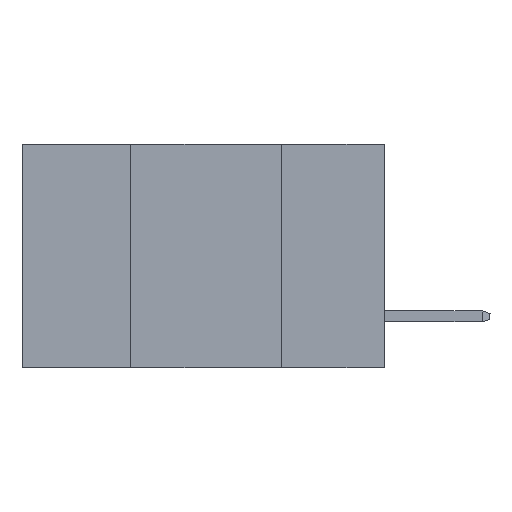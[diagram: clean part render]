
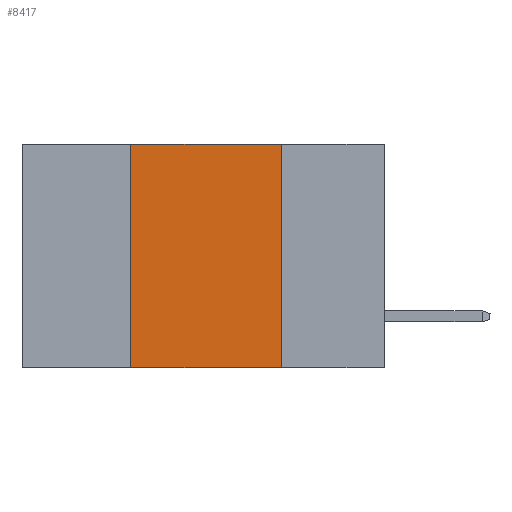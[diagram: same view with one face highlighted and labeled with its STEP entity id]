
A CAD part, left-side view. The second image highlights one B-rep face of the part: STEP entity #8417.
In plain terms, the highlighted planar face has unit normal (-1, 0, 0).
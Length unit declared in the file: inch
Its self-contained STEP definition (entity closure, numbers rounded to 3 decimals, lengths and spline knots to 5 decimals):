
#395 = DIRECTION ( 'NONE',  ( 0., 0., 1. ) ) ;
#570 = LINE ( 'NONE', #4150, #7495 ) ;
#981 = VECTOR ( 'NONE', #5233, 39.37008 ) ;
#1358 = EDGE_CURVE ( 'NONE', #10059, #4949, #4970, .T. ) ;
#1696 = LINE ( 'NONE', #1801, #981 ) ;
#1801 = CARTESIAN_POINT ( 'NONE',  ( 0., 0.6, 0. ) ) ;
#1817 = EDGE_CURVE ( 'NONE', #10059, #9994, #570, .T. ) ;
#1960 = ORIENTED_EDGE ( 'NONE', *, *, #1817, .F. ) ;
#2254 = EDGE_CURVE ( 'NONE', #6924, #4949, #11538, .T. ) ;
#2487 = DIRECTION ( 'NONE',  ( 0., -1., 0. ) ) ;
#2564 = CARTESIAN_POINT ( 'NONE',  ( 0., 0.17, -0.37 ) ) ;
#4150 = CARTESIAN_POINT ( 'NONE',  ( 0., 0.42, -0.37 ) ) ;
#4535 = CARTESIAN_POINT ( 'NONE',  ( 0., 0.42, 0. ) ) ;
#4606 = FACE_OUTER_BOUND ( 'NONE', #9052, .T. ) ;
#4664 = EDGE_CURVE ( 'NONE', #9994, #6924, #1696, .T. ) ;
#4949 = VERTEX_POINT ( 'NONE', #9545 ) ;
#4970 = LINE ( 'NONE', #6088, #8031 ) ;
#5233 = DIRECTION ( 'NONE',  ( 0., -1., 0. ) ) ;
#5314 = PLANE ( 'NONE',  #10304 ) ;
#6088 = CARTESIAN_POINT ( 'NONE',  ( 0., 0.6, -0.37 ) ) ;
#6427 = CARTESIAN_POINT ( 'NONE',  ( 0., 0.42, -0.37 ) ) ;
#6924 = VERTEX_POINT ( 'NONE', #9093 ) ;
#6939 = ORIENTED_EDGE ( 'NONE', *, *, #1358, .T. ) ;
#7211 = DIRECTION ( 'NONE',  ( 0., 0., -1. ) ) ;
#7314 = ORIENTED_EDGE ( 'NONE', *, *, #2254, .F. ) ;
#7495 = VECTOR ( 'NONE', #395, 39.37008 ) ;
#8031 = VECTOR ( 'NONE', #2487, 39.37008 ) ;
#8417 = ADVANCED_FACE ( 'NONE', ( #4606 ), #5314, .F. ) ;
#9052 = EDGE_LOOP ( 'NONE', ( #7314, #9212, #1960, #6939 ) ) ;
#9093 = CARTESIAN_POINT ( 'NONE',  ( 0., 0.17, 0. ) ) ;
#9212 = ORIENTED_EDGE ( 'NONE', *, *, #4664, .F. ) ;
#9545 = CARTESIAN_POINT ( 'NONE',  ( 0., 0.17, -0.37 ) ) ;
#9764 = DIRECTION ( 'NONE',  ( 0., 0., -1. ) ) ;
#9867 = CARTESIAN_POINT ( 'NONE',  ( 0., 0.6, 0. ) ) ;
#9994 = VERTEX_POINT ( 'NONE', #4535 ) ;
#10059 = VERTEX_POINT ( 'NONE', #6427 ) ;
#10304 = AXIS2_PLACEMENT_3D ( 'NONE', #9867, #10753, #7211 ) ;
#10536 = VECTOR ( 'NONE', #9764, 39.37008 ) ;
#10753 = DIRECTION ( 'NONE',  ( 1., 0., 0. ) ) ;
#11538 = LINE ( 'NONE', #2564, #10536 ) ;
